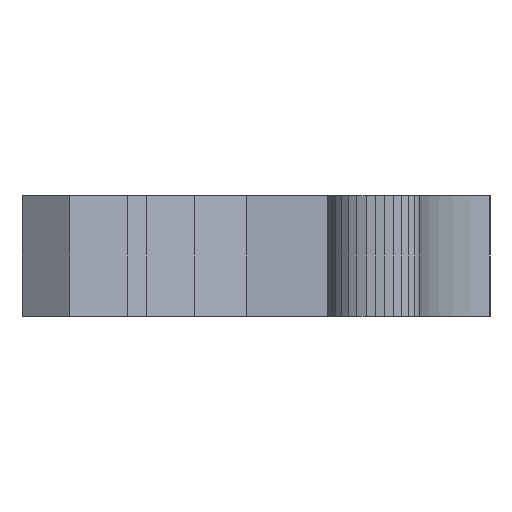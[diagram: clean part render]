
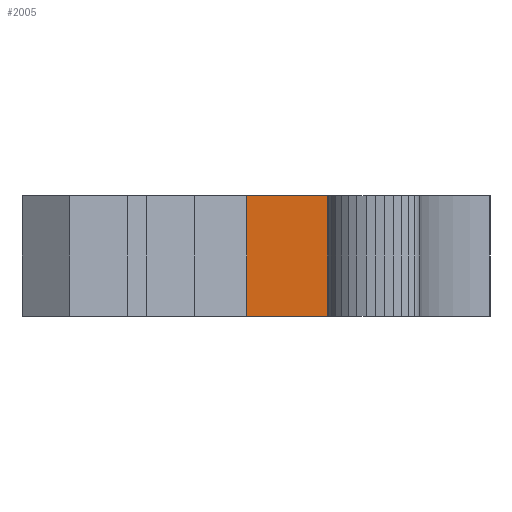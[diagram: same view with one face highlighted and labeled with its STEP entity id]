
A CAD part, front view. The second image highlights one B-rep face of the part: STEP entity #2005.
In plain terms, the highlighted planar face has unit normal (-0.016, -1, 0).
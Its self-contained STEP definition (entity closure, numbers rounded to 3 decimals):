
#1949=CARTESIAN_POINT('',(-5.709,30.373,0.0));
#1950=VERTEX_POINT('',#1949);
#1958=CARTESIAN_POINT('',(-5.709,30.373,10.0));
#1959=VERTEX_POINT('',#1958);
#1966=CARTESIAN_POINT('',(-5.709,30.373,0.0));
#1967=DIRECTION('',(0.0,0.0,1.0));
#1968=VECTOR('',#1967,10.0);
#1969=LINE('',#1966,#1968);
#1970=EDGE_CURVE('',#1950,#1959,#1969,.T.);
#1975=CARTESIAN_POINT('',(-12.883,30.486,0.0));
#1976=DIRECTION('',(-0.016,-1.,0.0));
#1977=DIRECTION('',(1.,-0.016,0.0));
#1978=AXIS2_PLACEMENT_3D('',#1975,#1976,#1977);
#1979=PLANE('',#1978);
#1980=CARTESIAN_POINT('',(-12.883,30.486,0.0));
#1981=VERTEX_POINT('',#1980);
#1982=CARTESIAN_POINT('',(-12.883,30.486,0.0));
#1983=DIRECTION('',(1.,-0.016,0.0));
#1984=VECTOR('',#1983,7.175);
#1985=LINE('',#1982,#1984);
#1986=EDGE_CURVE('',#1981,#1950,#1985,.T.);
#1987=ORIENTED_EDGE('',*,*,#1986,.T.);
#1988=ORIENTED_EDGE('',*,*,#1970,.T.);
#1989=CARTESIAN_POINT('',(-12.883,30.486,10.0));
#1990=VERTEX_POINT('',#1989);
#1991=CARTESIAN_POINT('',(-12.883,30.486,10.0));
#1992=DIRECTION('',(1.,-0.016,0.0));
#1993=VECTOR('',#1992,7.175);
#1994=LINE('',#1991,#1993);
#1995=EDGE_CURVE('',#1990,#1959,#1994,.T.);
#1996=ORIENTED_EDGE('',*,*,#1995,.F.);
#1997=CARTESIAN_POINT('',(-12.883,30.486,0.0));
#1998=DIRECTION('',(0.0,0.0,1.0));
#1999=VECTOR('',#1998,10.0);
#2000=LINE('',#1997,#1999);
#2001=EDGE_CURVE('',#1981,#1990,#2000,.T.);
#2002=ORIENTED_EDGE('',*,*,#2001,.F.);
#2003=EDGE_LOOP('',(#1987,#1988,#1996,#2002));
#2004=FACE_OUTER_BOUND('',#2003,.T.);
#2005=ADVANCED_FACE('',(#2004),#1979,.T.);
